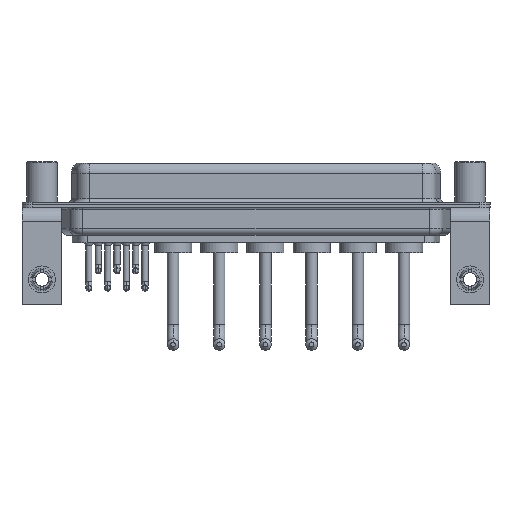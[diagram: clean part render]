
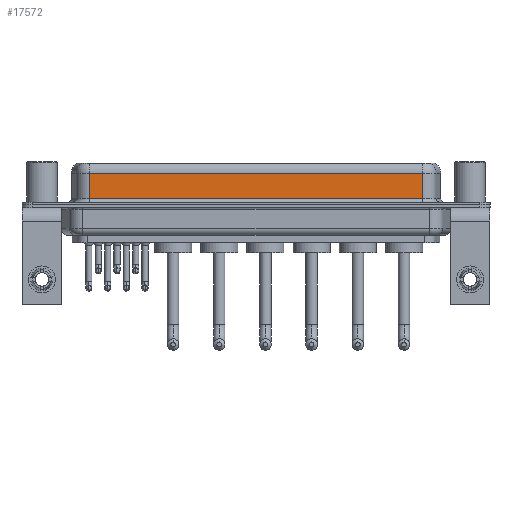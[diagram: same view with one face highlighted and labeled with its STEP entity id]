
A CAD part, front view. The second image highlights one B-rep face of the part: STEP entity #17572.
In plain terms, the highlighted planar face has unit normal (0, -1, 0).
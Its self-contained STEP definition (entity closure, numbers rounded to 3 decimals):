
#687 = CARTESIAN_POINT ( 'NONE',  ( 7.038, -3.95, 0.9 ) ) ;
#718 = VERTEX_POINT ( 'NONE', #687 ) ;
#1671 = PLANE ( 'NONE',  #6472 ) ;
#1708 = ORIENTED_EDGE ( 'NONE', *, *, #18803, .T. ) ;
#1879 = VECTOR ( 'NONE', #5973, 1000. ) ;
#2021 = CARTESIAN_POINT ( 'NONE',  ( 7.038, -3.95, 4.65 ) ) ;
#2182 = ORIENTED_EDGE ( 'NONE', *, *, #17383, .F. ) ;
#2787 = LINE ( 'NONE', #14774, #16793 ) ;
#4678 = EDGE_CURVE ( 'NONE', #7628, #718, #20325, .T. ) ;
#5767 = EDGE_LOOP ( 'NONE', ( #2182, #6838, #6736, #1708 ) ) ;
#5973 = DIRECTION ( 'NONE',  ( 0., 0., -1. ) ) ;
#6102 = VERTEX_POINT ( 'NONE', #20241 ) ;
#6472 = AXIS2_PLACEMENT_3D ( 'NONE', #13100, #8420, #18199 ) ;
#6736 = ORIENTED_EDGE ( 'NONE', *, *, #4678, .T. ) ;
#6838 = ORIENTED_EDGE ( 'NONE', *, *, #21417, .T. ) ;
#7038 = CARTESIAN_POINT ( 'NONE',  ( 56.462, -3.95, 4.65 ) ) ;
#7262 = VECTOR ( 'NONE', #21948, 1000. ) ;
#7529 = DIRECTION ( 'NONE',  ( 1., 0., 0. ) ) ;
#7628 = VERTEX_POINT ( 'NONE', #2021 ) ;
#8310 = FACE_OUTER_BOUND ( 'NONE', #5767, .T. ) ;
#8420 = DIRECTION ( 'NONE',  ( 0., 1., 0. ) ) ;
#8588 = LINE ( 'NONE', #7038, #7262 ) ;
#9893 = CARTESIAN_POINT ( 'NONE',  ( 7.038, -3.95, 6.4 ) ) ;
#13100 = CARTESIAN_POINT ( 'NONE',  ( 56.462, -3.95, 6.4 ) ) ;
#14622 = VECTOR ( 'NONE', #16641, 1000. ) ;
#14774 = CARTESIAN_POINT ( 'NONE',  ( 56.462, -3.95, 0.9 ) ) ;
#15687 = VERTEX_POINT ( 'NONE', #20561 ) ;
#16641 = DIRECTION ( 'NONE',  ( 0., 0., -1. ) ) ;
#16793 = VECTOR ( 'NONE', #7529, 1000. ) ;
#17383 = EDGE_CURVE ( 'NONE', #6102, #15687, #17667, .T. ) ;
#17572 = ADVANCED_FACE ( 'NONE', ( #8310 ), #1671, .F. ) ;
#17667 = LINE ( 'NONE', #21223, #1879 ) ;
#18199 = DIRECTION ( 'NONE',  ( 0., 0., 1. ) ) ;
#18803 = EDGE_CURVE ( 'NONE', #718, #15687, #2787, .T. ) ;
#20241 = CARTESIAN_POINT ( 'NONE',  ( 56.462, -3.95, 4.65 ) ) ;
#20325 = LINE ( 'NONE', #9893, #14622 ) ;
#20561 = CARTESIAN_POINT ( 'NONE',  ( 56.462, -3.95, 0.9 ) ) ;
#21223 = CARTESIAN_POINT ( 'NONE',  ( 56.462, -3.95, 6.4 ) ) ;
#21417 = EDGE_CURVE ( 'NONE', #6102, #7628, #8588, .T. ) ;
#21948 = DIRECTION ( 'NONE',  ( -1., 0., 0. ) ) ;
